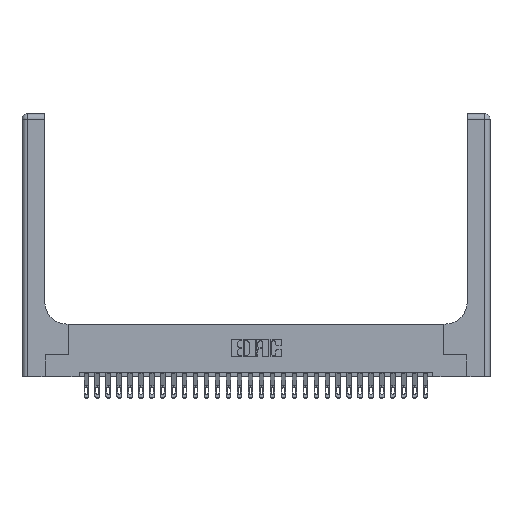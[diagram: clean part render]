
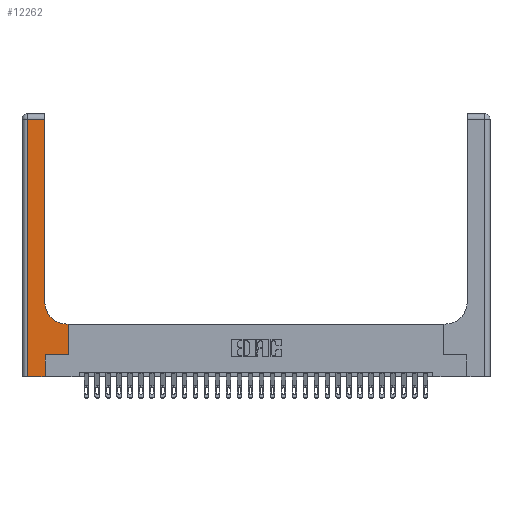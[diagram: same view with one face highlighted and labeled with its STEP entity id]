
A CAD part, top view. The second image highlights one B-rep face of the part: STEP entity #12262.
In plain terms, the highlighted planar face has unit normal (0, 0, 1).
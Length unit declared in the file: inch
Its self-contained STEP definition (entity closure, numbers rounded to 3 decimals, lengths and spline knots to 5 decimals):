
#481 = ORIENTED_EDGE ( 'NONE', *, *, #21221, .T. ) ;
#747 = VERTEX_POINT ( 'NONE', #4239 ) ;
#831 = CARTESIAN_POINT ( 'NONE',  ( 0.265, 0.25, 0.37 ) ) ;
#1101 = CARTESIAN_POINT ( 'NONE',  ( 0., 3., 0.37 ) ) ;
#1377 = PLANE ( 'NONE',  #26244 ) ;
#1556 = LINE ( 'NONE', #18055, #18013 ) ;
#1753 = CARTESIAN_POINT ( 'NONE',  ( 0.51, 0.6, 0.37 ) ) ;
#2094 = ORIENTED_EDGE ( 'NONE', *, *, #23576, .T. ) ;
#2199 = VERTEX_POINT ( 'NONE', #13056 ) ;
#3233 = DIRECTION ( 'NONE',  ( -1., 0., 0. ) ) ;
#3239 = CARTESIAN_POINT ( 'NONE',  ( 0.26, 0.85, 0.37 ) ) ;
#3487 = LINE ( 'NONE', #25146, #24330 ) ;
#3976 = CARTESIAN_POINT ( 'NONE',  ( 0.528, 0.25, 0.37 ) ) ;
#4239 = CARTESIAN_POINT ( 'NONE',  ( 0.528, 0.6, 0.37 ) ) ;
#4467 = VECTOR ( 'NONE', #26335, 39.37008 ) ;
#4762 = CARTESIAN_POINT ( 'NONE',  ( 0., 2.94, 0.37 ) ) ;
#5214 = LINE ( 'NONE', #8953, #11624 ) ;
#5526 = LINE ( 'NONE', #26651, #12610 ) ;
#6501 = DIRECTION ( 'NONE',  ( 0., -1., 0. ) ) ;
#6777 = FACE_OUTER_BOUND ( 'NONE', #19116, .T. ) ;
#6931 = DIRECTION ( 'NONE',  ( 0., 1., 0. ) ) ;
#7300 = LINE ( 'NONE', #4762, #23393 ) ;
#7305 = VECTOR ( 'NONE', #6501, 39.37008 ) ;
#7744 = VERTEX_POINT ( 'NONE', #3239 ) ;
#8315 = CARTESIAN_POINT ( 'NONE',  ( 0.51, 0.85, 0.37 ) ) ;
#8614 = EDGE_CURVE ( 'NONE', #2199, #21301, #7300, .T. ) ;
#8707 = ORIENTED_EDGE ( 'NONE', *, *, #24002, .T. ) ;
#8839 = ORIENTED_EDGE ( 'NONE', *, *, #20315, .T. ) ;
#8850 = CARTESIAN_POINT ( 'NONE',  ( 0.06, 0., 0.37 ) ) ;
#8953 = CARTESIAN_POINT ( 'NONE',  ( 0.265, 0.25, 0.37 ) ) ;
#9017 = ORIENTED_EDGE ( 'NONE', *, *, #22134, .T. ) ;
#9289 = CIRCLE ( 'NONE', #10986, 0.25 ) ;
#9920 = EDGE_CURVE ( 'NONE', #11130, #19070, #5214, .T. ) ;
#10113 = EDGE_CURVE ( 'NONE', #7744, #2199, #1556, .T. ) ;
#10944 = DIRECTION ( 'NONE',  ( 1., 0., 0. ) ) ;
#10986 = AXIS2_PLACEMENT_3D ( 'NONE', #8315, #23119, #27322 ) ;
#11130 = VERTEX_POINT ( 'NONE', #831 ) ;
#11624 = VECTOR ( 'NONE', #10944, 39.37008 ) ;
#11968 = CARTESIAN_POINT ( 'NONE',  ( 0.265, 0., 0.37 ) ) ;
#12202 = CARTESIAN_POINT ( 'NONE',  ( 0.06, 2.94, 0.37 ) ) ;
#12262 = ADVANCED_FACE ( 'NONE', ( #6777 ), #1377, .F. ) ;
#12610 = VECTOR ( 'NONE', #24512, 39.37008 ) ;
#13017 = ORIENTED_EDGE ( 'NONE', *, *, #15632, .T. ) ;
#13056 = CARTESIAN_POINT ( 'NONE',  ( 0.26, 2.94, 0.37 ) ) ;
#14593 = ORIENTED_EDGE ( 'NONE', *, *, #8614, .T. ) ;
#15265 = ORIENTED_EDGE ( 'NONE', *, *, #10113, .T. ) ;
#15632 = EDGE_CURVE ( 'NONE', #23764, #21974, #27300, .T. ) ;
#16118 = DIRECTION ( 'NONE',  ( 0., 0., -1. ) ) ;
#17501 = CARTESIAN_POINT ( 'NONE',  ( 0.06, 3., 0.37 ) ) ;
#18013 = VECTOR ( 'NONE', #26463, 39.37008 ) ;
#18055 = CARTESIAN_POINT ( 'NONE',  ( 0.26, 3., 0.37 ) ) ;
#19070 = VERTEX_POINT ( 'NONE', #3976 ) ;
#19116 = EDGE_LOOP ( 'NONE', ( #15265, #14593, #8839, #13017, #481, #19166, #8707, #9017, #2094 ) ) ;
#19166 = ORIENTED_EDGE ( 'NONE', *, *, #9920, .T. ) ;
#20315 = EDGE_CURVE ( 'NONE', #21301, #23764, #21743, .T. ) ;
#21045 = LINE ( 'NONE', #24010, #24722 ) ;
#21221 = EDGE_CURVE ( 'NONE', #21974, #11130, #21045, .T. ) ;
#21301 = VERTEX_POINT ( 'NONE', #12202 ) ;
#21743 = LINE ( 'NONE', #17501, #7305 ) ;
#21974 = VERTEX_POINT ( 'NONE', #11968 ) ;
#22134 = EDGE_CURVE ( 'NONE', #747, #26111, #3487, .T. ) ;
#23119 = DIRECTION ( 'NONE',  ( 0., 0., -1. ) ) ;
#23180 = DIRECTION ( 'NONE',  ( -1., 0., 0. ) ) ;
#23393 = VECTOR ( 'NONE', #24405, 39.37008 ) ;
#23576 = EDGE_CURVE ( 'NONE', #26111, #7744, #9289, .T. ) ;
#23764 = VERTEX_POINT ( 'NONE', #8850 ) ;
#24002 = EDGE_CURVE ( 'NONE', #19070, #747, #5526, .T. ) ;
#24010 = CARTESIAN_POINT ( 'NONE',  ( 0.265, 0., 0.37 ) ) ;
#24330 = VECTOR ( 'NONE', #23180, 39.37008 ) ;
#24405 = DIRECTION ( 'NONE',  ( -1., 0., 0. ) ) ;
#24512 = DIRECTION ( 'NONE',  ( 0., 1., 0. ) ) ;
#24722 = VECTOR ( 'NONE', #6931, 39.37008 ) ;
#25146 = CARTESIAN_POINT ( 'NONE',  ( 0.26, 0.6, 0.37 ) ) ;
#26111 = VERTEX_POINT ( 'NONE', #1753 ) ;
#26140 = CARTESIAN_POINT ( 'NONE',  ( 0., 0., 0.37 ) ) ;
#26244 = AXIS2_PLACEMENT_3D ( 'NONE', #1101, #16118, #3233 ) ;
#26335 = DIRECTION ( 'NONE',  ( 1., 0., 0. ) ) ;
#26463 = DIRECTION ( 'NONE',  ( 0., 1., 0. ) ) ;
#26651 = CARTESIAN_POINT ( 'NONE',  ( 0.528, 0.25, 0.37 ) ) ;
#27300 = LINE ( 'NONE', #26140, #4467 ) ;
#27322 = DIRECTION ( 'NONE',  ( 1., 0., 0. ) ) ;
